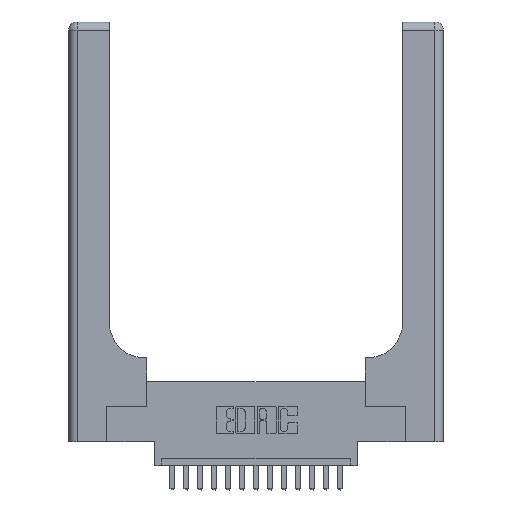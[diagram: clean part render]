
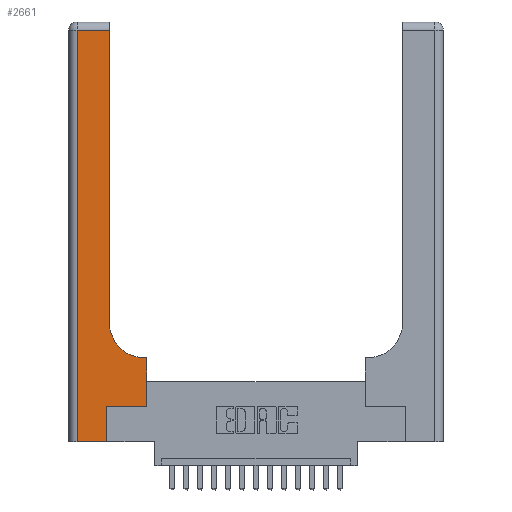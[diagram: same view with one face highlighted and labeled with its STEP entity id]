
A CAD part, top view. The second image highlights one B-rep face of the part: STEP entity #2661.
In plain terms, the highlighted planar face has unit normal (0, 0, 1).
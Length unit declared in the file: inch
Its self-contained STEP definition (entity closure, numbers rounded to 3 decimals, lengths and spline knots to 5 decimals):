
#21 = DIRECTION ( 'NONE',  ( -1., 0., 0. ) ) ;
#101 = CARTESIAN_POINT ( 'NONE',  ( 0.5585, 0.6, 0.37 ) ) ;
#135 = DIRECTION ( 'NONE',  ( 0., 0., -1. ) ) ;
#224 = VERTEX_POINT ( 'NONE', #2524 ) ;
#289 = VECTOR ( 'NONE', #15021, 39.37008 ) ;
#321 = PLANE ( 'NONE',  #2591 ) ;
#359 = DIRECTION ( 'NONE',  ( 0., -1., 0. ) ) ;
#693 = LINE ( 'NONE', #4747, #8765 ) ;
#794 = ORIENTED_EDGE ( 'NONE', *, *, #12974, .T. ) ;
#879 = CARTESIAN_POINT ( 'NONE',  ( 0.2915, 3., 0.37 ) ) ;
#1072 = CARTESIAN_POINT ( 'NONE',  ( 0.2915, 2.94, 0.37 ) ) ;
#1163 = LINE ( 'NONE', #10061, #6659 ) ;
#1340 = ORIENTED_EDGE ( 'NONE', *, *, #4268, .T. ) ;
#1493 = CARTESIAN_POINT ( 'NONE',  ( 0.5585, 0.25, 0.37 ) ) ;
#1572 = VECTOR ( 'NONE', #2012, 39.37008 ) ;
#1721 = EDGE_CURVE ( 'NONE', #10613, #12868, #12334, .T. ) ;
#2012 = DIRECTION ( 'NONE',  ( -1., 0., 0. ) ) ;
#2121 = LINE ( 'NONE', #1493, #17377 ) ;
#2502 = EDGE_CURVE ( 'NONE', #6095, #10639, #17364, .T. ) ;
#2524 = CARTESIAN_POINT ( 'NONE',  ( 0.06, 2.94, 0.37 ) ) ;
#2591 = AXIS2_PLACEMENT_3D ( 'NONE', #17958, #135, #3082 ) ;
#2661 = ADVANCED_FACE ( 'NONE', ( #9721 ), #321, .F. ) ;
#3082 = DIRECTION ( 'NONE',  ( -1., 0., 0. ) ) ;
#3639 = ORIENTED_EDGE ( 'NONE', *, *, #1721, .T. ) ;
#4268 = EDGE_CURVE ( 'NONE', #12868, #9641, #1163, .T. ) ;
#4747 = CARTESIAN_POINT ( 'NONE',  ( 0.06, 3., 0.37 ) ) ;
#6095 = VERTEX_POINT ( 'NONE', #16302 ) ;
#6659 = VECTOR ( 'NONE', #15989, 39.37008 ) ;
#7213 = ORIENTED_EDGE ( 'NONE', *, *, #17297, .T. ) ;
#7459 = DIRECTION ( 'NONE',  ( 0., 1., 0. ) ) ;
#7734 = CARTESIAN_POINT ( 'NONE',  ( 0.269, 0., 0.37 ) ) ;
#8765 = VECTOR ( 'NONE', #359, 39.37008 ) ;
#8853 = CARTESIAN_POINT ( 'NONE',  ( 0.2915, 0.6, 0.37 ) ) ;
#8854 = DIRECTION ( 'NONE',  ( 1., 0., 0. ) ) ;
#9087 = CARTESIAN_POINT ( 'NONE',  ( 0.2915, 0.85, 0.37 ) ) ;
#9191 = ORIENTED_EDGE ( 'NONE', *, *, #11783, .T. ) ;
#9326 = EDGE_CURVE ( 'NONE', #10639, #9379, #16051, .T. ) ;
#9379 = VERTEX_POINT ( 'NONE', #1072 ) ;
#9641 = VERTEX_POINT ( 'NONE', #10432 ) ;
#9721 = FACE_OUTER_BOUND ( 'NONE', #10146, .T. ) ;
#9737 = CARTESIAN_POINT ( 'NONE',  ( 0.269, 0., 0.37 ) ) ;
#9966 = ORIENTED_EDGE ( 'NONE', *, *, #9326, .T. ) ;
#10061 = CARTESIAN_POINT ( 'NONE',  ( 0.269, 0.25, 0.37 ) ) ;
#10146 = EDGE_LOOP ( 'NONE', ( #9966, #9191, #794, #7213, #3639, #1340, #17276, #14236, #17760 ) ) ;
#10432 = CARTESIAN_POINT ( 'NONE',  ( 0.5585, 0.25, 0.37 ) ) ;
#10613 = VERTEX_POINT ( 'NONE', #7734 ) ;
#10639 = VERTEX_POINT ( 'NONE', #9087 ) ;
#11357 = VECTOR ( 'NONE', #21, 39.37008 ) ;
#11748 = DIRECTION ( 'NONE',  ( 0., 0., -1. ) ) ;
#11783 = EDGE_CURVE ( 'NONE', #9379, #224, #12867, .T. ) ;
#12119 = VECTOR ( 'NONE', #14262, 39.37008 ) ;
#12334 = LINE ( 'NONE', #9737, #17213 ) ;
#12867 = LINE ( 'NONE', #15276, #1572 ) ;
#12868 = VERTEX_POINT ( 'NONE', #16143 ) ;
#12974 = EDGE_CURVE ( 'NONE', #224, #19130, #693, .T. ) ;
#13283 = CARTESIAN_POINT ( 'NONE',  ( 0., 0., 0.37 ) ) ;
#13628 = CARTESIAN_POINT ( 'NONE',  ( 0.06, 0., 0.37 ) ) ;
#14236 = ORIENTED_EDGE ( 'NONE', *, *, #18956, .T. ) ;
#14262 = DIRECTION ( 'NONE',  ( 0., 1., 0. ) ) ;
#14292 = VERTEX_POINT ( 'NONE', #101 ) ;
#14766 = LINE ( 'NONE', #8853, #11357 ) ;
#15021 = DIRECTION ( 'NONE',  ( 1., 0., 0. ) ) ;
#15276 = CARTESIAN_POINT ( 'NONE',  ( 0., 2.94, 0.37 ) ) ;
#15989 = DIRECTION ( 'NONE',  ( 1., 0., 0. ) ) ;
#16051 = LINE ( 'NONE', #879, #12119 ) ;
#16143 = CARTESIAN_POINT ( 'NONE',  ( 0.269, 0.25, 0.37 ) ) ;
#16180 = CARTESIAN_POINT ( 'NONE',  ( 0.5415, 0.85, 0.37 ) ) ;
#16302 = CARTESIAN_POINT ( 'NONE',  ( 0.5415, 0.6, 0.37 ) ) ;
#16961 = DIRECTION ( 'NONE',  ( 0., 1., 0. ) ) ;
#17213 = VECTOR ( 'NONE', #16961, 39.37008 ) ;
#17276 = ORIENTED_EDGE ( 'NONE', *, *, #18380, .T. ) ;
#17297 = EDGE_CURVE ( 'NONE', #19130, #10613, #18777, .T. ) ;
#17364 = CIRCLE ( 'NONE', #18787, 0.25 ) ;
#17377 = VECTOR ( 'NONE', #7459, 39.37008 ) ;
#17760 = ORIENTED_EDGE ( 'NONE', *, *, #2502, .T. ) ;
#17958 = CARTESIAN_POINT ( 'NONE',  ( 0., 3., 0.37 ) ) ;
#18380 = EDGE_CURVE ( 'NONE', #9641, #14292, #2121, .T. ) ;
#18777 = LINE ( 'NONE', #13283, #289 ) ;
#18787 = AXIS2_PLACEMENT_3D ( 'NONE', #16180, #11748, #8854 ) ;
#18956 = EDGE_CURVE ( 'NONE', #14292, #6095, #14766, .T. ) ;
#19130 = VERTEX_POINT ( 'NONE', #13628 ) ;
